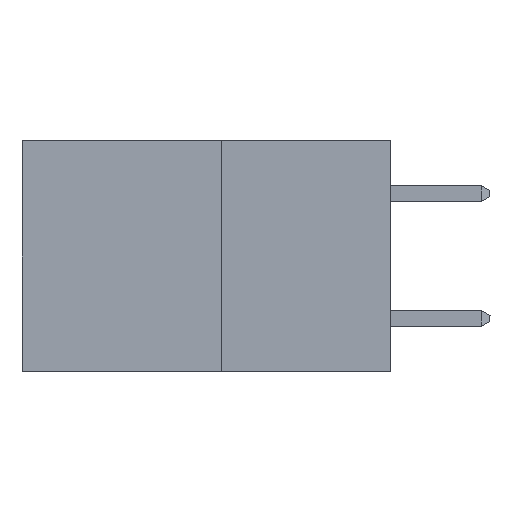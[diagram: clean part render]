
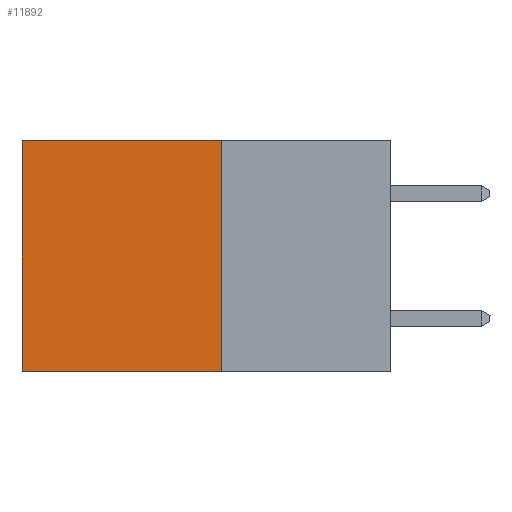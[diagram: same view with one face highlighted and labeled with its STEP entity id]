
A CAD part, left-side view. The second image highlights one B-rep face of the part: STEP entity #11892.
In plain terms, the highlighted planar face has unit normal (-1, 0, 0).
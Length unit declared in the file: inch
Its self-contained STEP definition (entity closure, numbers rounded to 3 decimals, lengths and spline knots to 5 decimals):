
#632 = EDGE_CURVE ( 'NONE', #22489, #23125, #19208, .T. ) ;
#3773 = LINE ( 'NONE', #20338, #8395 ) ;
#4637 = CARTESIAN_POINT ( 'NONE',  ( 0.277, 0.27, 0. ) ) ;
#5535 = CARTESIAN_POINT ( 'NONE',  ( 0.277, 0.27, -0.37 ) ) ;
#6750 = EDGE_LOOP ( 'NONE', ( #19093, #17588, #11428, #12492 ) ) ;
#7025 = DIRECTION ( 'NONE',  ( 1., 0., 0. ) ) ;
#7523 = DIRECTION ( 'NONE',  ( 0., 1., 0. ) ) ;
#8395 = VECTOR ( 'NONE', #22261, 39.37008 ) ;
#10548 = DIRECTION ( 'NONE',  ( 0., 1., 0. ) ) ;
#11377 = CARTESIAN_POINT ( 'NONE',  ( 0.277, 0.59, -0.37 ) ) ;
#11428 = ORIENTED_EDGE ( 'NONE', *, *, #14772, .F. ) ;
#11431 = VERTEX_POINT ( 'NONE', #13458 ) ;
#11892 = ADVANCED_FACE ( 'NONE', ( #16212 ), #24513, .F. ) ;
#12492 = ORIENTED_EDGE ( 'NONE', *, *, #12814, .T. ) ;
#12814 = EDGE_CURVE ( 'NONE', #19026, #22489, #20764, .T. ) ;
#12900 = CARTESIAN_POINT ( 'NONE',  ( 0.277, 0.59, -0.37 ) ) ;
#13458 = CARTESIAN_POINT ( 'NONE',  ( 0.277, 0.27, -0.37 ) ) ;
#14558 = VECTOR ( 'NONE', #7523, 39.37008 ) ;
#14772 = EDGE_CURVE ( 'NONE', #19026, #11431, #3773, .T. ) ;
#15552 = VECTOR ( 'NONE', #10548, 39.37008 ) ;
#16212 = FACE_OUTER_BOUND ( 'NONE', #6750, .T. ) ;
#17588 = ORIENTED_EDGE ( 'NONE', *, *, #20590, .F. ) ;
#18564 = AXIS2_PLACEMENT_3D ( 'NONE', #18732, #7025, #20712 ) ;
#18732 = CARTESIAN_POINT ( 'NONE',  ( 0.277, 0.27, -0.37 ) ) ;
#19026 = VERTEX_POINT ( 'NONE', #4637 ) ;
#19093 = ORIENTED_EDGE ( 'NONE', *, *, #632, .T. ) ;
#19208 = LINE ( 'NONE', #12900, #23763 ) ;
#20101 = DIRECTION ( 'NONE',  ( 0., 0., -1. ) ) ;
#20338 = CARTESIAN_POINT ( 'NONE',  ( 0.277, 0.27, -0.37 ) ) ;
#20590 = EDGE_CURVE ( 'NONE', #11431, #23125, #24924, .T. ) ;
#20712 = DIRECTION ( 'NONE',  ( 0., 0., -1. ) ) ;
#20764 = LINE ( 'NONE', #24205, #15552 ) ;
#22261 = DIRECTION ( 'NONE',  ( 0., 0., -1. ) ) ;
#22489 = VERTEX_POINT ( 'NONE', #22936 ) ;
#22936 = CARTESIAN_POINT ( 'NONE',  ( 0.277, 0.59, 0. ) ) ;
#23125 = VERTEX_POINT ( 'NONE', #11377 ) ;
#23763 = VECTOR ( 'NONE', #20101, 39.37008 ) ;
#24205 = CARTESIAN_POINT ( 'NONE',  ( 0.277, 0.27, 0. ) ) ;
#24513 = PLANE ( 'NONE',  #18564 ) ;
#24924 = LINE ( 'NONE', #5535, #14558 ) ;
